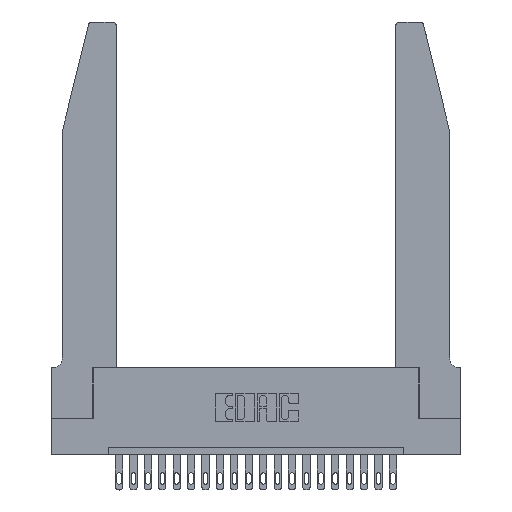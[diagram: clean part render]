
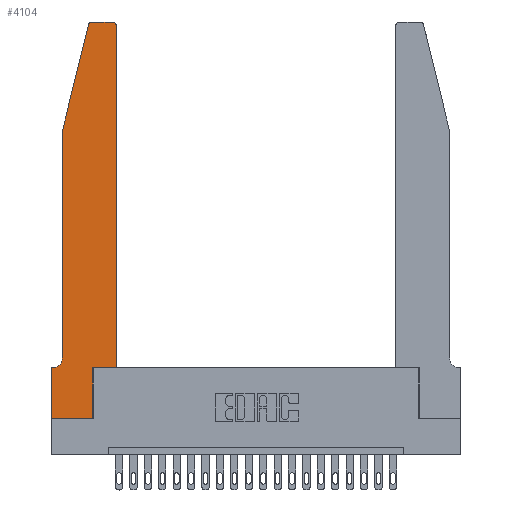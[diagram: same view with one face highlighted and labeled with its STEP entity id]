
A CAD part, top view. The second image highlights one B-rep face of the part: STEP entity #4104.
In plain terms, the highlighted planar face has unit normal (0, 0, 1).
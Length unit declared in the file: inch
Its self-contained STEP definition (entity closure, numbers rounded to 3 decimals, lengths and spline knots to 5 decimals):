
#226 = AXIS2_PLACEMENT_3D ( 'NONE', #1920, #6974, #3475 ) ;
#445 = EDGE_CURVE ( 'NONE', #11140, #2130, #13643, .T. ) ;
#511 = DIRECTION ( 'NONE',  ( 1., 0., 0. ) ) ;
#627 = CARTESIAN_POINT ( 'NONE',  ( 0.0755, 0.42, 0.37 ) ) ;
#744 = EDGE_CURVE ( 'NONE', #1961, #5777, #4069, .T. ) ;
#927 = ORIENTED_EDGE ( 'NONE', *, *, #6642, .T. ) ;
#973 = CARTESIAN_POINT ( 'NONE',  ( 0.0755, 0.35, 0.37 ) ) ;
#1267 = LINE ( 'NONE', #12683, #19325 ) ;
#1392 = LINE ( 'NONE', #11961, #14835 ) ;
#1413 = ORIENTED_EDGE ( 'NONE', *, *, #17293, .T. ) ;
#1578 = CARTESIAN_POINT ( 'NONE',  ( 0.2865, 0., 0.37 ) ) ;
#1920 = CARTESIAN_POINT ( 'NONE',  ( 0.284, 2.72, 0.37 ) ) ;
#1945 = DIRECTION ( 'NONE',  ( 0., -1., 0. ) ) ;
#1961 = VERTEX_POINT ( 'NONE', #22649 ) ;
#2130 = VERTEX_POINT ( 'NONE', #13102 ) ;
#2211 = VECTOR ( 'NONE', #16394, 39.37008 ) ;
#2246 = PLANE ( 'NONE',  #5539 ) ;
#2321 = CARTESIAN_POINT ( 'NONE',  ( 0.0055, 0.35, 0.37 ) ) ;
#2340 = ORIENTED_EDGE ( 'NONE', *, *, #12449, .T. ) ;
#2462 = EDGE_CURVE ( 'NONE', #4870, #6112, #1267, .T. ) ;
#2531 = CARTESIAN_POINT ( 'NONE',  ( 0.0755, 2., 0.37 ) ) ;
#2563 = CARTESIAN_POINT ( 'NONE',  ( 0.25487, 2.72718, 0.37 ) ) ;
#3397 = DIRECTION ( 'NONE',  ( 1., 0., 0. ) ) ;
#3475 = DIRECTION ( 'NONE',  ( 1., 0., 0. ) ) ;
#3531 = CARTESIAN_POINT ( 'NONE',  ( 0., 0., 0.37 ) ) ;
#3543 = VECTOR ( 'NONE', #9066, 39.37008 ) ;
#3986 = CARTESIAN_POINT ( 'NONE',  ( 0.0055, 0.42, 0.37 ) ) ;
#4069 = LINE ( 'NONE', #21135, #12278 ) ;
#4104 = ADVANCED_FACE ( 'NONE', ( #11925 ), #2246, .T. ) ;
#4125 = VERTEX_POINT ( 'NONE', #7443 ) ;
#4138 = AXIS2_PLACEMENT_3D ( 'NONE', #9415, #5837, #511 ) ;
#4148 = VERTEX_POINT ( 'NONE', #2321 ) ;
#4870 = VERTEX_POINT ( 'NONE', #2531 ) ;
#5377 = EDGE_CURVE ( 'NONE', #19135, #9621, #6369, .T. ) ;
#5474 = DIRECTION ( 'NONE',  ( 1., 0., 0. ) ) ;
#5539 = AXIS2_PLACEMENT_3D ( 'NONE', #10915, #12839, #5474 ) ;
#5777 = VERTEX_POINT ( 'NONE', #8394 ) ;
#5837 = DIRECTION ( 'NONE',  ( 0., 0., 1. ) ) ;
#6112 = VERTEX_POINT ( 'NONE', #627 ) ;
#6369 = CIRCLE ( 'NONE', #226, 0.03 ) ;
#6596 = DIRECTION ( 'NONE',  ( -0.239, -0.971, 0. ) ) ;
#6642 = EDGE_CURVE ( 'NONE', #5777, #4125, #21908, .T. ) ;
#6974 = DIRECTION ( 'NONE',  ( 0., 0., 1. ) ) ;
#7143 = ORIENTED_EDGE ( 'NONE', *, *, #5377, .T. ) ;
#7320 = VECTOR ( 'NONE', #9322, 39.37008 ) ;
#7360 = ORIENTED_EDGE ( 'NONE', *, *, #445, .T. ) ;
#7443 = CARTESIAN_POINT ( 'NONE',  ( 0.4505, 2.72, 0.37 ) ) ;
#7479 = VERTEX_POINT ( 'NONE', #1578 ) ;
#7933 = VECTOR ( 'NONE', #20174, 39.37008 ) ;
#8394 = CARTESIAN_POINT ( 'NONE',  ( 0.4505, 0.35, 0.37 ) ) ;
#8500 = LINE ( 'NONE', #9060, #2211 ) ;
#9060 = CARTESIAN_POINT ( 'NONE',  ( 0.2865, 0.35, 0.37 ) ) ;
#9066 = DIRECTION ( 'NONE',  ( 0., -1., 0. ) ) ;
#9101 = DIRECTION ( 'NONE',  ( 0., 0., -1. ) ) ;
#9322 = DIRECTION ( 'NONE',  ( -1., 0., 0. ) ) ;
#9401 = DIRECTION ( 'NONE',  ( -1., 0., 0. ) ) ;
#9415 = CARTESIAN_POINT ( 'NONE',  ( 0.4205, 2.72, 0.37 ) ) ;
#9545 = CARTESIAN_POINT ( 'NONE',  ( 0.4505, 0.35, 0.37 ) ) ;
#9619 = CIRCLE ( 'NONE', #17233, 0.07 ) ;
#9621 = VERTEX_POINT ( 'NONE', #2563 ) ;
#10121 = ORIENTED_EDGE ( 'NONE', *, *, #20696, .T. ) ;
#10915 = CARTESIAN_POINT ( 'NONE',  ( 0., 0.35, 0.37 ) ) ;
#11088 = ORIENTED_EDGE ( 'NONE', *, *, #18448, .T. ) ;
#11140 = VERTEX_POINT ( 'NONE', #11396 ) ;
#11396 = CARTESIAN_POINT ( 'NONE',  ( 0., 0.35, 0.37 ) ) ;
#11746 = ORIENTED_EDGE ( 'NONE', *, *, #2462, .T. ) ;
#11925 = FACE_OUTER_BOUND ( 'NONE', #20276, .T. ) ;
#11961 = CARTESIAN_POINT ( 'NONE',  ( 0.0755, 2., 0.37 ) ) ;
#12278 = VECTOR ( 'NONE', #3397, 39.37008 ) ;
#12449 = EDGE_CURVE ( 'NONE', #2130, #7479, #17030, .T. ) ;
#12479 = CIRCLE ( 'NONE', #4138, 0.03 ) ;
#12683 = CARTESIAN_POINT ( 'NONE',  ( 0.0755, 2., 0.37 ) ) ;
#12839 = DIRECTION ( 'NONE',  ( 0., 0., 1. ) ) ;
#13102 = CARTESIAN_POINT ( 'NONE',  ( 0., 0., 0.37 ) ) ;
#13236 = CARTESIAN_POINT ( 'NONE',  ( 0.4205, 2.75, 0.37 ) ) ;
#13256 = EDGE_CURVE ( 'NONE', #7479, #1961, #8500, .T. ) ;
#13265 = ORIENTED_EDGE ( 'NONE', *, *, #744, .T. ) ;
#13643 = LINE ( 'NONE', #18222, #3543 ) ;
#13914 = DIRECTION ( 'NONE',  ( 1., 0., 0. ) ) ;
#14260 = EDGE_CURVE ( 'NONE', #6112, #4148, #9619, .T. ) ;
#14835 = VECTOR ( 'NONE', #6596, 39.37008 ) ;
#15198 = VECTOR ( 'NONE', #18261, 39.37008 ) ;
#16394 = DIRECTION ( 'NONE',  ( 0., 1., 0. ) ) ;
#17030 = LINE ( 'NONE', #3531, #18126 ) ;
#17233 = AXIS2_PLACEMENT_3D ( 'NONE', #3986, #9101, #9401 ) ;
#17293 = EDGE_CURVE ( 'NONE', #19257, #19135, #21287, .T. ) ;
#17808 = CARTESIAN_POINT ( 'NONE',  ( 0.2605, 2.75, 0.37 ) ) ;
#18126 = VECTOR ( 'NONE', #13914, 39.37008 ) ;
#18222 = CARTESIAN_POINT ( 'NONE',  ( 0., 0., 0.37 ) ) ;
#18261 = DIRECTION ( 'NONE',  ( -1., 0., 0. ) ) ;
#18448 = EDGE_CURVE ( 'NONE', #4125, #19257, #12479, .T. ) ;
#18584 = EDGE_CURVE ( 'NONE', #4148, #11140, #19849, .T. ) ;
#19135 = VERTEX_POINT ( 'NONE', #19794 ) ;
#19190 = ORIENTED_EDGE ( 'NONE', *, *, #18584, .T. ) ;
#19257 = VERTEX_POINT ( 'NONE', #13236 ) ;
#19325 = VECTOR ( 'NONE', #1945, 39.37008 ) ;
#19554 = ORIENTED_EDGE ( 'NONE', *, *, #13256, .T. ) ;
#19794 = CARTESIAN_POINT ( 'NONE',  ( 0.284, 2.75, 0.37 ) ) ;
#19849 = LINE ( 'NONE', #973, #15198 ) ;
#20174 = DIRECTION ( 'NONE',  ( 0., 1., 0. ) ) ;
#20276 = EDGE_LOOP ( 'NONE', ( #1413, #7143, #10121, #11746, #20940, #19190, #7360, #2340, #19554, #13265, #927, #11088 ) ) ;
#20696 = EDGE_CURVE ( 'NONE', #9621, #4870, #1392, .T. ) ;
#20940 = ORIENTED_EDGE ( 'NONE', *, *, #14260, .T. ) ;
#21135 = CARTESIAN_POINT ( 'NONE',  ( 0.4505, 0.35, 0.37 ) ) ;
#21287 = LINE ( 'NONE', #17808, #7320 ) ;
#21908 = LINE ( 'NONE', #9545, #7933 ) ;
#22649 = CARTESIAN_POINT ( 'NONE',  ( 0.2865, 0.35, 0.37 ) ) ;
